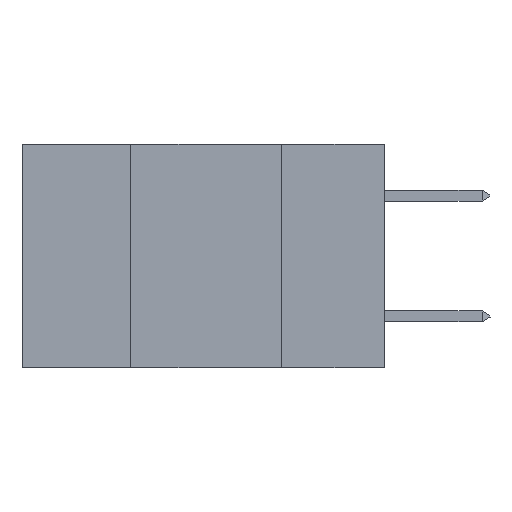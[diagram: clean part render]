
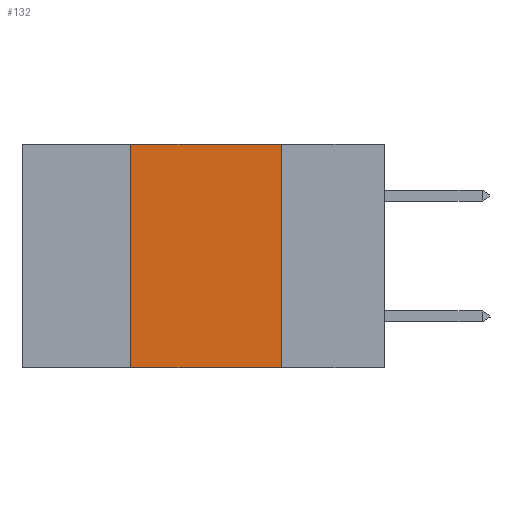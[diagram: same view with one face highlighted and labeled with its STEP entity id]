
A CAD part, left-side view. The second image highlights one B-rep face of the part: STEP entity #132.
In plain terms, the highlighted planar face has unit normal (-1, 0, 0).
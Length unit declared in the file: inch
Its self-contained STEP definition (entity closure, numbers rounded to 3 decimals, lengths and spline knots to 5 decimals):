
#70 = ORIENTED_EDGE ( 'NONE', *, *, #7789, .F. ) ;
#132 = ADVANCED_FACE ( 'NONE', ( #5672 ), #3006, .F. ) ;
#401 = CARTESIAN_POINT ( 'NONE',  ( 0., 0.42, 0. ) ) ;
#790 = DIRECTION ( 'NONE',  ( 1., 0., 0. ) ) ;
#936 = EDGE_CURVE ( 'NONE', #3528, #6927, #12785, .T. ) ;
#983 = EDGE_LOOP ( 'NONE', ( #6531, #70, #3608, #7299 ) ) ;
#3006 = PLANE ( 'NONE',  #9644 ) ;
#3062 = DIRECTION ( 'NONE',  ( 0., 0., -1. ) ) ;
#3528 = VERTEX_POINT ( 'NONE', #8175 ) ;
#3608 = ORIENTED_EDGE ( 'NONE', *, *, #13252, .F. ) ;
#4196 = VECTOR ( 'NONE', #13530, 39.37008 ) ;
#4574 = VECTOR ( 'NONE', #13016, 39.37008 ) ;
#4844 = VECTOR ( 'NONE', #5127, 39.37008 ) ;
#5127 = DIRECTION ( 'NONE',  ( 0., -1., 0. ) ) ;
#5219 = CARTESIAN_POINT ( 'NONE',  ( 0., 0.17, 0. ) ) ;
#5672 = FACE_OUTER_BOUND ( 'NONE', #983, .T. ) ;
#6076 = CARTESIAN_POINT ( 'NONE',  ( 0., 0.17, -0.37 ) ) ;
#6387 = CARTESIAN_POINT ( 'NONE',  ( 0., 0.6, 0. ) ) ;
#6531 = ORIENTED_EDGE ( 'NONE', *, *, #13090, .F. ) ;
#6650 = CARTESIAN_POINT ( 'NONE',  ( 0., 0.6, -0.37 ) ) ;
#6927 = VERTEX_POINT ( 'NONE', #6076 ) ;
#7299 = ORIENTED_EDGE ( 'NONE', *, *, #936, .T. ) ;
#7789 = EDGE_CURVE ( 'NONE', #12261, #9032, #12713, .T. ) ;
#8012 = CARTESIAN_POINT ( 'NONE',  ( 0., 0.17, 0. ) ) ;
#8175 = CARTESIAN_POINT ( 'NONE',  ( 0., 0.42, -0.37 ) ) ;
#8562 = VECTOR ( 'NONE', #10576, 39.37008 ) ;
#8783 = CARTESIAN_POINT ( 'NONE',  ( 0., 0.42, 0. ) ) ;
#9032 = VERTEX_POINT ( 'NONE', #8012 ) ;
#9644 = AXIS2_PLACEMENT_3D ( 'NONE', #6387, #790, #3062 ) ;
#10463 = CARTESIAN_POINT ( 'NONE',  ( 0., 0.6, 0. ) ) ;
#10576 = DIRECTION ( 'NONE',  ( 0., 0., -1. ) ) ;
#11438 = LINE ( 'NONE', #5219, #8562 ) ;
#12261 = VERTEX_POINT ( 'NONE', #401 ) ;
#12474 = LINE ( 'NONE', #8783, #4196 ) ;
#12713 = LINE ( 'NONE', #10463, #4844 ) ;
#12785 = LINE ( 'NONE', #6650, #4574 ) ;
#13016 = DIRECTION ( 'NONE',  ( 0., -1., 0. ) ) ;
#13090 = EDGE_CURVE ( 'NONE', #9032, #6927, #11438, .T. ) ;
#13252 = EDGE_CURVE ( 'NONE', #3528, #12261, #12474, .T. ) ;
#13530 = DIRECTION ( 'NONE',  ( 0., 0., 1. ) ) ;
